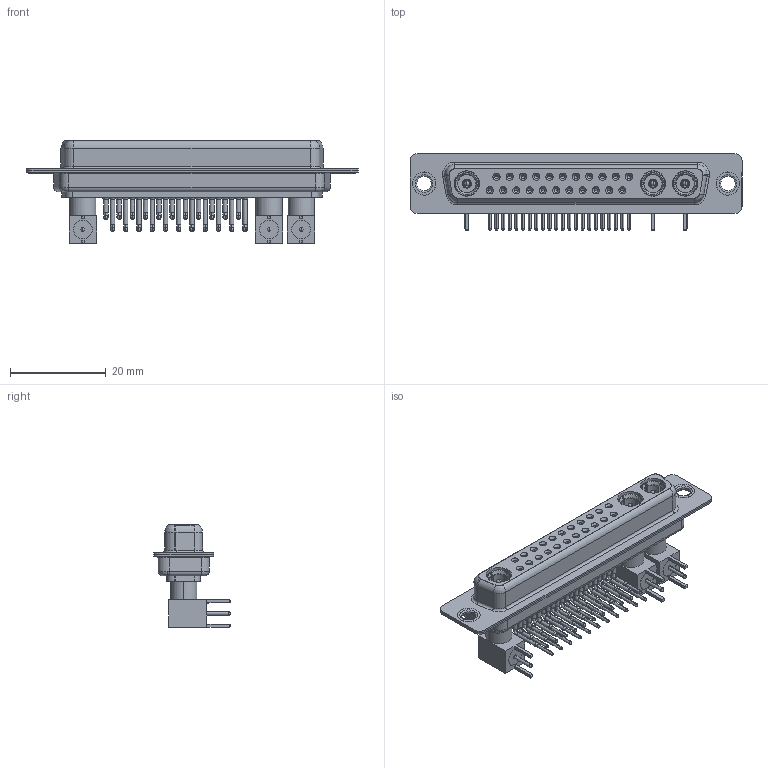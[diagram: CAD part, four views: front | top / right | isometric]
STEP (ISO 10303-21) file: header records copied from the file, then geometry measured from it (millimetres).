
FILE_DESCRIPTION (( 'STEP AP203' ), '1' );
FILE_NAME ('630-25W3240-5N1.STEP', '2022-06-07T03:33:01', ( '' ), ( '' ), 'SwSTEP 2.0', 'SolidWorks 2020', '' );
FILE_SCHEMA (( 'CONFIG_CONTROL_DESIGN' ));
Length unit declared in the file: millimetre
Products named in the file (16): Co-Ax Plug Assy_RA; 630Combo Housing_25W3; Locking Collar; Pin_RA; Insulator RA Pin; Co-Ax Plug_RA PC Tail; 630Combo Shell Rear_37 Contacts; RA Back Shell; Insulator Pin_Straight PC Tail; 630-25W3240-5N1; 630Combo Contact Row 1; 630Combo Shell Front_37 Contacts; 630Combo Thru Hole Rivet; 630Combo Contact Row 2
Assembly tree (48 placements, depth 3):
  630-25W3240-5N1
    630Combo Housing_25W3
    630Combo Shell Front_37 Contacts
    630Combo Shell Rear_37 Contacts
    630Combo Thru Hole Rivet  x2
    Co-Ax Plug Assy_RA
      Co-Ax Plug_RA PC Tail
      Insulator Pin_Straight PC Tail
      Pin_RA
      Locking Collar
      RA Back Shell
      Insulator RA Pin
    Co-Ax Plug Assy_RA
      Co-Ax Plug_RA PC Tail
      Insulator Pin_Straight PC Tail
      Pin_RA
      Locking Collar
      RA Back Shell
      Insulator RA Pin
    Co-Ax Plug Assy_RA
      Co-Ax Plug_RA PC Tail
      Insulator Pin_Straight PC Tail
      Pin_RA
      Locking Collar
      RA Back Shell
      Insulator RA Pin
    630Combo Contact Row 1  x11
    630Combo Contact Row 2  x11
Bounding box: 69.4 x 16 x 21.41 mm (x, y, z)
Volume: 6095.7 mm3; surface area: 14434.8 mm2
Topology: 45 solids, 45 shells, 1923 faces, 4776 edges, 2994 vertices
Faces by surface type: cylinder 822, plane 598, cone 317, bspline 91, torus 83, sphere 12
Entity records: 25631 total; most frequent: CARTESIAN_POINT 4368, DIRECTION 4333, ORIENTED_EDGE 3596, AXIS2_PLACEMENT_3D 1800, EDGE_CURVE 1798, VERTEX_POINT 1142, CIRCLE 978, EDGE_LOOP 946
